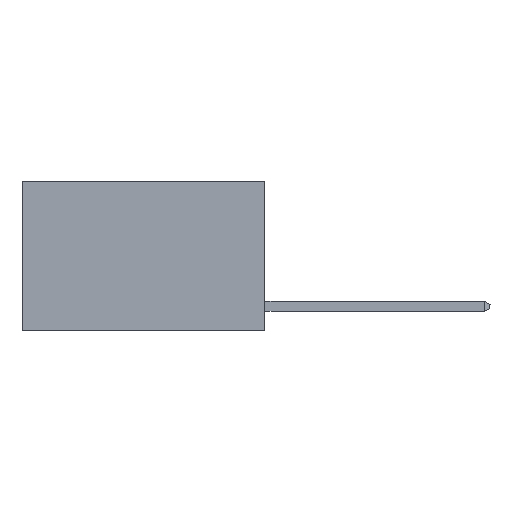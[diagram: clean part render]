
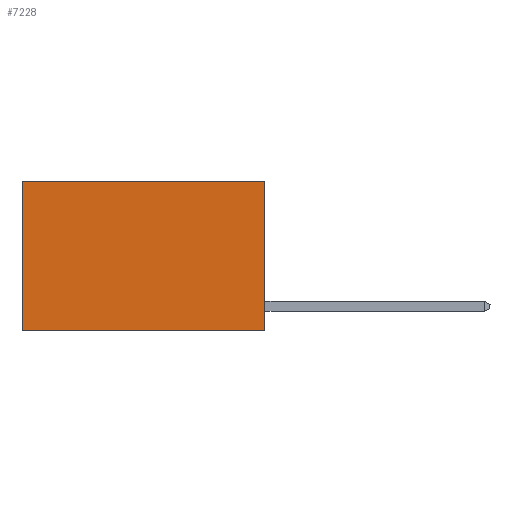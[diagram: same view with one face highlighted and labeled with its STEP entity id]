
A CAD part, left-side view. The second image highlights one B-rep face of the part: STEP entity #7228.
In plain terms, the highlighted planar face has unit normal (-1, 0, 0).
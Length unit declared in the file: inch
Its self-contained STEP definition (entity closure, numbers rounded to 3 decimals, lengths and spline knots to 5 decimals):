
#240 = CARTESIAN_POINT ( 'NONE',  ( 0.2625, 0., 0. ) ) ;
#412 = CARTESIAN_POINT ( 'NONE',  ( 0.2625, 0.6, 0. ) ) ;
#604 = DIRECTION ( 'NONE',  ( 1., 0., 0. ) ) ;
#1686 = VERTEX_POINT ( 'NONE', #412 ) ;
#2673 = LINE ( 'NONE', #240, #12648 ) ;
#3730 = DIRECTION ( 'NONE',  ( 0., 0., -1. ) ) ;
#4030 = LINE ( 'NONE', #12493, #10470 ) ;
#4438 = VERTEX_POINT ( 'NONE', #11120 ) ;
#5595 = ORIENTED_EDGE ( 'NONE', *, *, #12241, .T. ) ;
#6474 = ORIENTED_EDGE ( 'NONE', *, *, #7907, .F. ) ;
#7228 = ADVANCED_FACE ( 'NONE', ( #7451 ), #13257, .F. ) ;
#7278 = VECTOR ( 'NONE', #3730, 39.37008 ) ;
#7451 = FACE_OUTER_BOUND ( 'NONE', #13804, .T. ) ;
#7907 = EDGE_CURVE ( 'NONE', #11983, #17935, #18270, .T. ) ;
#7958 = AXIS2_PLACEMENT_3D ( 'NONE', #10359, #604, #16077 ) ;
#8545 = CARTESIAN_POINT ( 'NONE',  ( 0.2625, 0., -0.37 ) ) ;
#9753 = DIRECTION ( 'NONE',  ( 0., 0., -1. ) ) ;
#9820 = DIRECTION ( 'NONE',  ( 0., 1., 0. ) ) ;
#10317 = ORIENTED_EDGE ( 'NONE', *, *, #11662, .T. ) ;
#10359 = CARTESIAN_POINT ( 'NONE',  ( 0.2625, 0., 0. ) ) ;
#10470 = VECTOR ( 'NONE', #9753, 39.37008 ) ;
#10793 = LINE ( 'NONE', #13590, #7278 ) ;
#11120 = CARTESIAN_POINT ( 'NONE',  ( 0.2625, 0., 0. ) ) ;
#11598 = DIRECTION ( 'NONE',  ( 0., 1., 0. ) ) ;
#11662 = EDGE_CURVE ( 'NONE', #4438, #1686, #2673, .T. ) ;
#11983 = VERTEX_POINT ( 'NONE', #8545 ) ;
#12241 = EDGE_CURVE ( 'NONE', #1686, #17935, #10793, .T. ) ;
#12493 = CARTESIAN_POINT ( 'NONE',  ( 0.2625, 0., 0. ) ) ;
#12559 = CARTESIAN_POINT ( 'NONE',  ( 0.2625, 0., -0.37 ) ) ;
#12648 = VECTOR ( 'NONE', #11598, 39.37008 ) ;
#13257 = PLANE ( 'NONE',  #7958 ) ;
#13590 = CARTESIAN_POINT ( 'NONE',  ( 0.2625, 0.6, 0. ) ) ;
#13715 = EDGE_CURVE ( 'NONE', #4438, #11983, #4030, .T. ) ;
#13804 = EDGE_LOOP ( 'NONE', ( #5595, #6474, #16924, #10317 ) ) ;
#14996 = CARTESIAN_POINT ( 'NONE',  ( 0.2625, 0.6, -0.37 ) ) ;
#16077 = DIRECTION ( 'NONE',  ( 0., 0., -1. ) ) ;
#16389 = VECTOR ( 'NONE', #9820, 39.37008 ) ;
#16924 = ORIENTED_EDGE ( 'NONE', *, *, #13715, .F. ) ;
#17935 = VERTEX_POINT ( 'NONE', #14996 ) ;
#18270 = LINE ( 'NONE', #12559, #16389 ) ;
